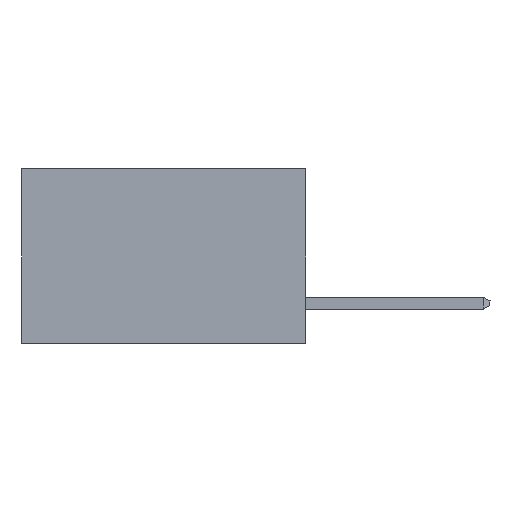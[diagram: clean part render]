
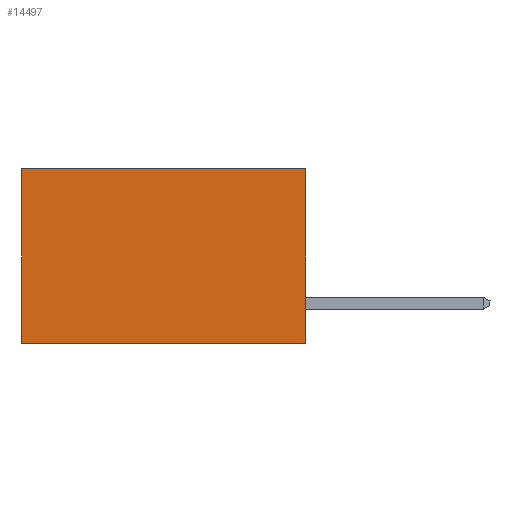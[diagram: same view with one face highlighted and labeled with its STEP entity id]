
A CAD part, left-side view. The second image highlights one B-rep face of the part: STEP entity #14497.
In plain terms, the highlighted planar face has unit normal (-1, 0, 0).
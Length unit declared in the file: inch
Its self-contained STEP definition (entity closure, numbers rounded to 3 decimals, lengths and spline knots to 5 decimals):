
#100 = CARTESIAN_POINT ( 'NONE',  ( 0.2615, 0.6, -0.37 ) ) ;
#831 = CARTESIAN_POINT ( 'NONE',  ( 0.2615, 0., -0.37 ) ) ;
#923 = CARTESIAN_POINT ( 'NONE',  ( 0.2615, 0., 0. ) ) ;
#1029 = LINE ( 'NONE', #18181, #19067 ) ;
#1350 = EDGE_CURVE ( 'NONE', #15959, #18776, #1029, .T. ) ;
#3010 = CARTESIAN_POINT ( 'NONE',  ( 0.2615, 0.6, 0. ) ) ;
#3539 = EDGE_CURVE ( 'NONE', #18776, #5473, #12255, .T. ) ;
#4853 = ORIENTED_EDGE ( 'NONE', *, *, #1350, .F. ) ;
#5473 = VERTEX_POINT ( 'NONE', #22951 ) ;
#8258 = FACE_OUTER_BOUND ( 'NONE', #9815, .T. ) ;
#9652 = VERTEX_POINT ( 'NONE', #3010 ) ;
#9815 = EDGE_LOOP ( 'NONE', ( #16642, #10714, #4853, #23023 ) ) ;
#10714 = ORIENTED_EDGE ( 'NONE', *, *, #3539, .F. ) ;
#11033 = VECTOR ( 'NONE', #12734, 39.37008 ) ;
#12255 = LINE ( 'NONE', #14059, #16308 ) ;
#12734 = DIRECTION ( 'NONE',  ( 0., 0., -1. ) ) ;
#13402 = DIRECTION ( 'NONE',  ( 0., 1., 0. ) ) ;
#14059 = CARTESIAN_POINT ( 'NONE',  ( 0.2615, 0., -0.37 ) ) ;
#14497 = ADVANCED_FACE ( 'NONE', ( #8258 ), #16883, .F. ) ;
#15848 = DIRECTION ( 'NONE',  ( 0., 0., -1. ) ) ;
#15959 = VERTEX_POINT ( 'NONE', #923 ) ;
#16041 = EDGE_CURVE ( 'NONE', #9652, #5473, #20175, .T. ) ;
#16190 = DIRECTION ( 'NONE',  ( 0., 1., 0. ) ) ;
#16308 = VECTOR ( 'NONE', #13402, 39.37008 ) ;
#16336 = CARTESIAN_POINT ( 'NONE',  ( 0.2615, 0., 0. ) ) ;
#16642 = ORIENTED_EDGE ( 'NONE', *, *, #16041, .T. ) ;
#16787 = DIRECTION ( 'NONE',  ( 0., 0., -1. ) ) ;
#16812 = DIRECTION ( 'NONE',  ( 1., 0., 0. ) ) ;
#16883 = PLANE ( 'NONE',  #21551 ) ;
#17648 = CARTESIAN_POINT ( 'NONE',  ( 0.2615, 0., -0.37 ) ) ;
#17962 = EDGE_CURVE ( 'NONE', #15959, #9652, #19597, .T. ) ;
#18181 = CARTESIAN_POINT ( 'NONE',  ( 0.2615, 0., -0.37 ) ) ;
#18572 = VECTOR ( 'NONE', #16190, 39.37008 ) ;
#18776 = VERTEX_POINT ( 'NONE', #831 ) ;
#19067 = VECTOR ( 'NONE', #15848, 39.37008 ) ;
#19597 = LINE ( 'NONE', #16336, #18572 ) ;
#20175 = LINE ( 'NONE', #100, #11033 ) ;
#21551 = AXIS2_PLACEMENT_3D ( 'NONE', #17648, #16812, #16787 ) ;
#22951 = CARTESIAN_POINT ( 'NONE',  ( 0.2615, 0.6, -0.37 ) ) ;
#23023 = ORIENTED_EDGE ( 'NONE', *, *, #17962, .T. ) ;
